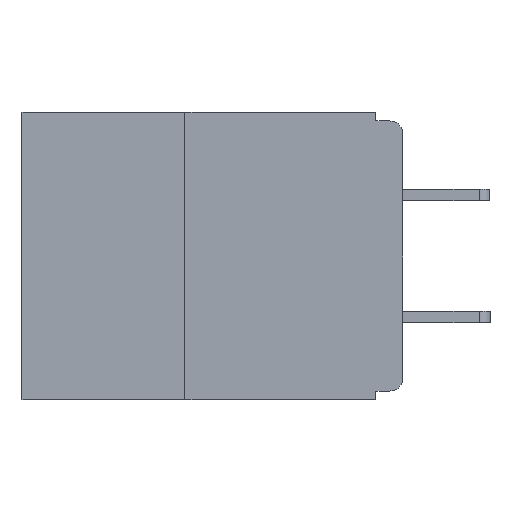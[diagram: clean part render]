
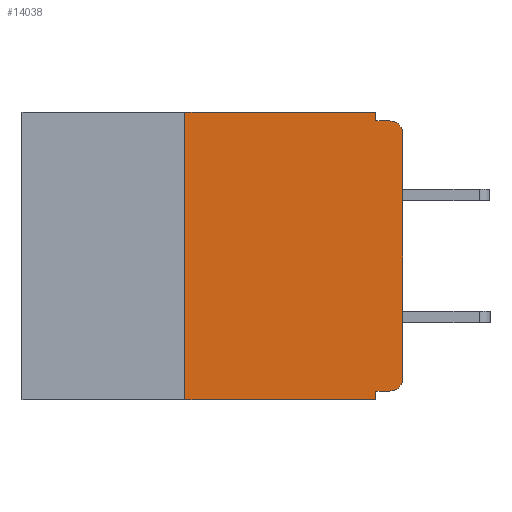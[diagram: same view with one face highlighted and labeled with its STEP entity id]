
A CAD part, left-side view. The second image highlights one B-rep face of the part: STEP entity #14038.
In plain terms, the highlighted planar face has unit normal (-1, 0, 0).
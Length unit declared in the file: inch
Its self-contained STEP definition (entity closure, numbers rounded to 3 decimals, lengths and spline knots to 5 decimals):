
#570 = CARTESIAN_POINT ( 'NONE',  ( 0., 0.25, -0.33 ) ) ;
#969 = ORIENTED_EDGE ( 'NONE', *, *, #6611, .F. ) ;
#1402 = VECTOR ( 'NONE', #18491, 39.37008 ) ;
#1800 = VERTEX_POINT ( 'NONE', #31919 ) ;
#2140 = CARTESIAN_POINT ( 'NONE',  ( 0., 0.031, -0.33 ) ) ;
#2185 = CARTESIAN_POINT ( 'NONE',  ( 0., 0.031, -0.01 ) ) ;
#2521 = DIRECTION ( 'NONE',  ( 0., 0., -1. ) ) ;
#4309 = CARTESIAN_POINT ( 'NONE',  ( 0., 0., -0.01 ) ) ;
#4506 = ORIENTED_EDGE ( 'NONE', *, *, #16236, .F. ) ;
#5084 = ORIENTED_EDGE ( 'NONE', *, *, #13001, .F. ) ;
#5103 = CARTESIAN_POINT ( 'NONE',  ( 0., 0.031, 0. ) ) ;
#5180 = AXIS2_PLACEMENT_3D ( 'NONE', #11431, #29013, #14014 ) ;
#6291 = ORIENTED_EDGE ( 'NONE', *, *, #14047, .T. ) ;
#6348 = LINE ( 'NONE', #4309, #19156 ) ;
#6566 = CARTESIAN_POINT ( 'NONE',  ( 0., 0.031, -0.32 ) ) ;
#6611 = EDGE_CURVE ( 'NONE', #30866, #19640, #18055, .T. ) ;
#6886 = AXIS2_PLACEMENT_3D ( 'NONE', #11318, #13898, #31350 ) ;
#7231 = VECTOR ( 'NONE', #13695, 39.37008 ) ;
#8157 = AXIS2_PLACEMENT_3D ( 'NONE', #8207, #25870, #10739 ) ;
#8207 = CARTESIAN_POINT ( 'NONE',  ( 0., 0.015, -0.025 ) ) ;
#8310 = ORIENTED_EDGE ( 'NONE', *, *, #10956, .T. ) ;
#8627 = VECTOR ( 'NONE', #27024, 39.37008 ) ;
#8870 = LINE ( 'NONE', #28251, #21577 ) ;
#10122 = ORIENTED_EDGE ( 'NONE', *, *, #29000, .F. ) ;
#10174 = CARTESIAN_POINT ( 'NONE',  ( 0., 0.031, -0.33 ) ) ;
#10196 = LINE ( 'NONE', #29509, #22873 ) ;
#10739 = DIRECTION ( 'NONE',  ( 0., 0., -1. ) ) ;
#10740 = CIRCLE ( 'NONE', #8157, 0.015 ) ;
#10956 = EDGE_CURVE ( 'NONE', #1800, #13459, #10740, .T. ) ;
#11318 = CARTESIAN_POINT ( 'NONE',  ( 0., 0.437, 0. ) ) ;
#11431 = CARTESIAN_POINT ( 'NONE',  ( 0., 0.015, -0.305 ) ) ;
#13001 = EDGE_CURVE ( 'NONE', #14009, #30866, #30241, .T. ) ;
#13121 = VERTEX_POINT ( 'NONE', #2185 ) ;
#13459 = VERTEX_POINT ( 'NONE', #28829 ) ;
#13695 = DIRECTION ( 'NONE',  ( 0., 0., 1. ) ) ;
#13788 = CARTESIAN_POINT ( 'NONE',  ( 0., 0.015, -0.32 ) ) ;
#13898 = DIRECTION ( 'NONE',  ( 1., 0., 0. ) ) ;
#14009 = VERTEX_POINT ( 'NONE', #13788 ) ;
#14014 = DIRECTION ( 'NONE',  ( 0., 0., -1. ) ) ;
#14038 = ADVANCED_FACE ( 'NONE', ( #18920 ), #26432, .F. ) ;
#14047 = EDGE_CURVE ( 'NONE', #14009, #20130, #18146, .T. ) ;
#15542 = EDGE_LOOP ( 'NONE', ( #20877, #8310, #10122, #31143, #26541, #4506, #19966, #969, #5084, #6291 ) ) ;
#15873 = LINE ( 'NONE', #15955, #1402 ) ;
#15955 = CARTESIAN_POINT ( 'NONE',  ( 0., 0.437, 0. ) ) ;
#16236 = EDGE_CURVE ( 'NONE', #20447, #19785, #20769, .T. ) ;
#16321 = CARTESIAN_POINT ( 'NONE',  ( 0., 0.25, -0.33 ) ) ;
#16458 = VERTEX_POINT ( 'NONE', #31872 ) ;
#18055 = LINE ( 'NONE', #2140, #30450 ) ;
#18146 = CIRCLE ( 'NONE', #5180, 0.015 ) ;
#18491 = DIRECTION ( 'NONE',  ( 0., -1., 0. ) ) ;
#18920 = FACE_OUTER_BOUND ( 'NONE', #15542, .T. ) ;
#19156 = VECTOR ( 'NONE', #19612, 39.37008 ) ;
#19503 = CARTESIAN_POINT ( 'NONE',  ( 0., 0., -0.32 ) ) ;
#19612 = DIRECTION ( 'NONE',  ( 0., -1., 0. ) ) ;
#19640 = VERTEX_POINT ( 'NONE', #10174 ) ;
#19785 = VERTEX_POINT ( 'NONE', #23348 ) ;
#19966 = ORIENTED_EDGE ( 'NONE', *, *, #25273, .T. ) ;
#20130 = VERTEX_POINT ( 'NONE', #32086 ) ;
#20433 = EDGE_CURVE ( 'NONE', #19785, #16458, #15873, .T. ) ;
#20447 = VERTEX_POINT ( 'NONE', #570 ) ;
#20769 = LINE ( 'NONE', #16321, #7231 ) ;
#20877 = ORIENTED_EDGE ( 'NONE', *, *, #26817, .T. ) ;
#21577 = VECTOR ( 'NONE', #30707, 39.37008 ) ;
#22873 = VECTOR ( 'NONE', #31932, 39.37008 ) ;
#23348 = CARTESIAN_POINT ( 'NONE',  ( 0., 0.25, 0. ) ) ;
#24102 = VECTOR ( 'NONE', #2521, 39.37008 ) ;
#25273 = EDGE_CURVE ( 'NONE', #20447, #19640, #10196, .T. ) ;
#25870 = DIRECTION ( 'NONE',  ( -1., 0., 0. ) ) ;
#26432 = PLANE ( 'NONE',  #6886 ) ;
#26541 = ORIENTED_EDGE ( 'NONE', *, *, #20433, .F. ) ;
#26817 = EDGE_CURVE ( 'NONE', #20130, #1800, #8870, .T. ) ;
#27024 = DIRECTION ( 'NONE',  ( 0., 1., 0. ) ) ;
#27521 = DIRECTION ( 'NONE',  ( 0., 0., -1. ) ) ;
#28251 = CARTESIAN_POINT ( 'NONE',  ( 0., 0., 0. ) ) ;
#28829 = CARTESIAN_POINT ( 'NONE',  ( 0., 0.015, -0.01 ) ) ;
#29000 = EDGE_CURVE ( 'NONE', #13121, #13459, #6348, .T. ) ;
#29013 = DIRECTION ( 'NONE',  ( -1., 0., 0. ) ) ;
#29509 = CARTESIAN_POINT ( 'NONE',  ( 0., 0.437, -0.33 ) ) ;
#30241 = LINE ( 'NONE', #19503, #8627 ) ;
#30450 = VECTOR ( 'NONE', #27521, 39.37008 ) ;
#30609 = LINE ( 'NONE', #5103, #24102 ) ;
#30707 = DIRECTION ( 'NONE',  ( 0., 0., 1. ) ) ;
#30866 = VERTEX_POINT ( 'NONE', #6566 ) ;
#31143 = ORIENTED_EDGE ( 'NONE', *, *, #31150, .F. ) ;
#31150 = EDGE_CURVE ( 'NONE', #16458, #13121, #30609, .T. ) ;
#31350 = DIRECTION ( 'NONE',  ( 0., 0., -1. ) ) ;
#31872 = CARTESIAN_POINT ( 'NONE',  ( 0., 0.031, 0. ) ) ;
#31919 = CARTESIAN_POINT ( 'NONE',  ( 0., 0., -0.025 ) ) ;
#31932 = DIRECTION ( 'NONE',  ( 0., -1., 0. ) ) ;
#32086 = CARTESIAN_POINT ( 'NONE',  ( 0., 0., -0.305 ) ) ;
